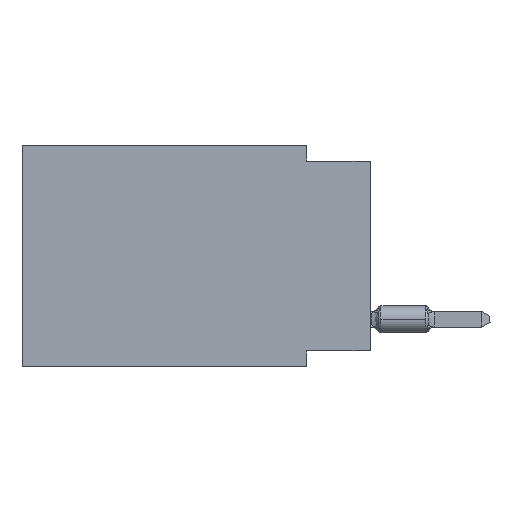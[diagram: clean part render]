
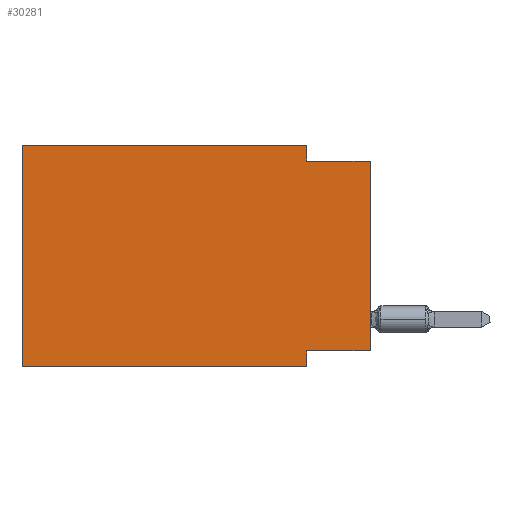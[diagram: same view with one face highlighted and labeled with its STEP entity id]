
A CAD part, left-side view. The second image highlights one B-rep face of the part: STEP entity #30281.
In plain terms, the highlighted planar face has unit normal (-1, 0, 0).
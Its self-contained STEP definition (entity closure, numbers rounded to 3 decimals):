
#384 = ORIENTED_EDGE ( 'NONE', *, *, #16119, .T. ) ;
#789 = AXIS2_PLACEMENT_3D ( 'NONE', #26626, #25804, #35681 ) ;
#1642 = CARTESIAN_POINT ( 'NONE',  ( 0., 2.54, -8.255 ) ) ;
#1913 = VERTEX_POINT ( 'NONE', #36353 ) ;
#2442 = VERTEX_POINT ( 'NONE', #8759 ) ;
#3923 = CARTESIAN_POINT ( 'NONE',  ( 0., 0., -8.255 ) ) ;
#5009 = LINE ( 'NONE', #5203, #29065 ) ;
#5203 = CARTESIAN_POINT ( 'NONE',  ( 0., 2.54, 0. ) ) ;
#5243 = CARTESIAN_POINT ( 'NONE',  ( 0., 13.97, 0. ) ) ;
#7060 = VERTEX_POINT ( 'NONE', #28672 ) ;
#8000 = ORIENTED_EDGE ( 'NONE', *, *, #14249, .F. ) ;
#8331 = PLANE ( 'NONE',  #789 ) ;
#8759 = CARTESIAN_POINT ( 'NONE',  ( 0., 2.54, -8.89 ) ) ;
#8833 = LINE ( 'NONE', #12435, #9752 ) ;
#9084 = VECTOR ( 'NONE', #18072, 1000. ) ;
#9472 = VERTEX_POINT ( 'NONE', #14374 ) ;
#9707 = VECTOR ( 'NONE', #23924, 1000. ) ;
#9752 = VECTOR ( 'NONE', #12229, 1000. ) ;
#9901 = LINE ( 'NONE', #31787, #26409 ) ;
#9971 = LINE ( 'NONE', #23902, #20616 ) ;
#10638 = VECTOR ( 'NONE', #22391, 1000. ) ;
#12229 = DIRECTION ( 'NONE',  ( 0., -1., 0. ) ) ;
#12435 = CARTESIAN_POINT ( 'NONE',  ( 0., 0., -0.635 ) ) ;
#13215 = DIRECTION ( 'NONE',  ( 0., 1., 0. ) ) ;
#13278 = VERTEX_POINT ( 'NONE', #28801 ) ;
#13953 = ORIENTED_EDGE ( 'NONE', *, *, #33852, .F. ) ;
#14033 = DIRECTION ( 'NONE',  ( 0., 0., -1. ) ) ;
#14117 = EDGE_CURVE ( 'NONE', #9472, #22205, #39189, .T. ) ;
#14249 = EDGE_CURVE ( 'NONE', #13278, #9472, #25236, .T. ) ;
#14366 = FACE_OUTER_BOUND ( 'NONE', #25387, .T. ) ;
#14374 = CARTESIAN_POINT ( 'NONE',  ( 0., 13.97, 0. ) ) ;
#16119 = EDGE_CURVE ( 'NONE', #24301, #1913, #9971, .T. ) ;
#16207 = LINE ( 'NONE', #28470, #36172 ) ;
#18072 = DIRECTION ( 'NONE',  ( 0., 0., 1. ) ) ;
#19578 = LINE ( 'NONE', #28427, #10638 ) ;
#19664 = ORIENTED_EDGE ( 'NONE', *, *, #38056, .F. ) ;
#20338 = CARTESIAN_POINT ( 'NONE',  ( 0., 2.54, 0. ) ) ;
#20616 = VECTOR ( 'NONE', #33530, 1000. ) ;
#21503 = EDGE_CURVE ( 'NONE', #7060, #1913, #8833, .T. ) ;
#22205 = VERTEX_POINT ( 'NONE', #20338 ) ;
#22391 = DIRECTION ( 'NONE',  ( 0., -1., 0. ) ) ;
#23902 = CARTESIAN_POINT ( 'NONE',  ( 0., 0., 0. ) ) ;
#23924 = DIRECTION ( 'NONE',  ( 0., -1., 0. ) ) ;
#24301 = VERTEX_POINT ( 'NONE', #3923 ) ;
#25236 = LINE ( 'NONE', #37506, #9084 ) ;
#25387 = EDGE_LOOP ( 'NONE', ( #384, #39283, #35374, #31133, #8000, #38194, #19664, #13953 ) ) ;
#25804 = DIRECTION ( 'NONE',  ( 1., 0., 0. ) ) ;
#26409 = VECTOR ( 'NONE', #34206, 1000. ) ;
#26626 = CARTESIAN_POINT ( 'NONE',  ( 0., 13.97, 0. ) ) ;
#27319 = EDGE_CURVE ( 'NONE', #13278, #2442, #19578, .T. ) ;
#28427 = CARTESIAN_POINT ( 'NONE',  ( 0., 13.97, -8.89 ) ) ;
#28470 = CARTESIAN_POINT ( 'NONE',  ( 0., 0., -8.255 ) ) ;
#28672 = CARTESIAN_POINT ( 'NONE',  ( 0., 2.54, -0.635 ) ) ;
#28801 = CARTESIAN_POINT ( 'NONE',  ( 0., 13.97, -8.89 ) ) ;
#29065 = VECTOR ( 'NONE', #14033, 1000. ) ;
#30281 = ADVANCED_FACE ( 'NONE', ( #14366 ), #8331, .F. ) ;
#31133 = ORIENTED_EDGE ( 'NONE', *, *, #14117, .F. ) ;
#31787 = CARTESIAN_POINT ( 'NONE',  ( 0., 2.54, -8.89 ) ) ;
#33488 = EDGE_CURVE ( 'NONE', #22205, #7060, #5009, .T. ) ;
#33530 = DIRECTION ( 'NONE',  ( 0., 0., 1. ) ) ;
#33852 = EDGE_CURVE ( 'NONE', #24301, #36965, #16207, .T. ) ;
#34206 = DIRECTION ( 'NONE',  ( 0., 0., -1. ) ) ;
#35374 = ORIENTED_EDGE ( 'NONE', *, *, #33488, .F. ) ;
#35681 = DIRECTION ( 'NONE',  ( 0., 0., -1. ) ) ;
#36172 = VECTOR ( 'NONE', #13215, 1000. ) ;
#36353 = CARTESIAN_POINT ( 'NONE',  ( 0., 0., -0.635 ) ) ;
#36965 = VERTEX_POINT ( 'NONE', #1642 ) ;
#37506 = CARTESIAN_POINT ( 'NONE',  ( 0., 13.97, 0. ) ) ;
#38056 = EDGE_CURVE ( 'NONE', #36965, #2442, #9901, .T. ) ;
#38194 = ORIENTED_EDGE ( 'NONE', *, *, #27319, .T. ) ;
#39189 = LINE ( 'NONE', #5243, #9707 ) ;
#39283 = ORIENTED_EDGE ( 'NONE', *, *, #21503, .F. ) ;
